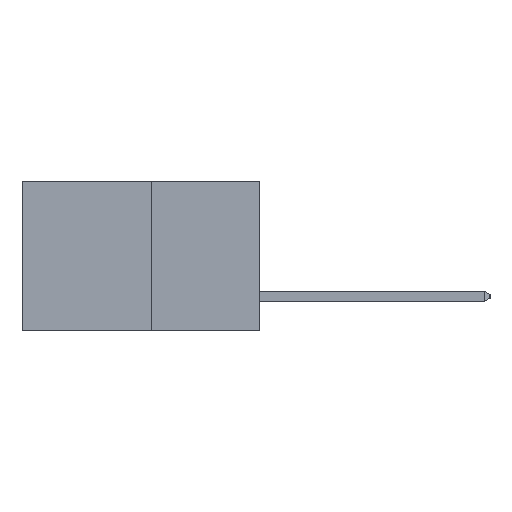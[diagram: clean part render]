
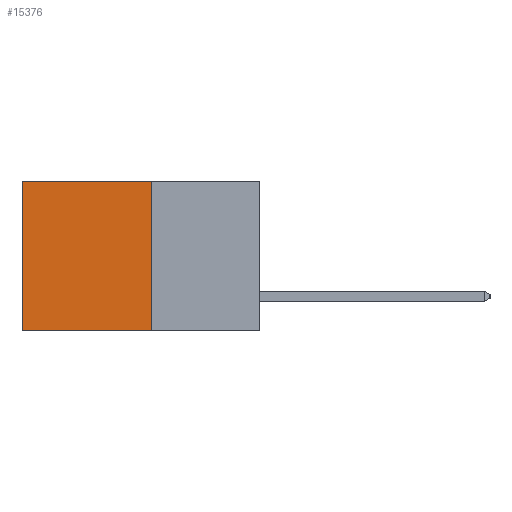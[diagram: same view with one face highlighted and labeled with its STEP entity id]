
A CAD part, left-side view. The second image highlights one B-rep face of the part: STEP entity #15376.
In plain terms, the highlighted planar face has unit normal (-1, 0, 0).
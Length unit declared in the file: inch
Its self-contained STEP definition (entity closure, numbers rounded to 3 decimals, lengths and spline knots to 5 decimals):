
#462 = DIRECTION ( 'NONE',  ( 1., 0., 0. ) ) ;
#981 = FACE_OUTER_BOUND ( 'NONE', #1252, .T. ) ;
#1162 = ORIENTED_EDGE ( 'NONE', *, *, #2322, .F. ) ;
#1252 = EDGE_LOOP ( 'NONE', ( #25020, #1162, #8642, #13474 ) ) ;
#1768 = EDGE_CURVE ( 'NONE', #18095, #10047, #10120, .T. ) ;
#2322 = EDGE_CURVE ( 'NONE', #16905, #10047, #8441, .T. ) ;
#2835 = DIRECTION ( 'NONE',  ( 0., 1., 0. ) ) ;
#3759 = CARTESIAN_POINT ( 'NONE',  ( 0.277, 0.27, -0.37 ) ) ;
#3883 = CARTESIAN_POINT ( 'NONE',  ( 0.277, 0.59, -0.37 ) ) ;
#4670 = VECTOR ( 'NONE', #23691, 39.37008 ) ;
#6234 = CARTESIAN_POINT ( 'NONE',  ( 0.277, 0.27, -0.37 ) ) ;
#6694 = VECTOR ( 'NONE', #22803, 39.37008 ) ;
#8441 = LINE ( 'NONE', #6234, #13174 ) ;
#8642 = ORIENTED_EDGE ( 'NONE', *, *, #23552, .F. ) ;
#8658 = CARTESIAN_POINT ( 'NONE',  ( 0.277, 0.59, -0.37 ) ) ;
#8874 = CARTESIAN_POINT ( 'NONE',  ( 0.277, 0.27, 0. ) ) ;
#9482 = VECTOR ( 'NONE', #9560, 39.37008 ) ;
#9560 = DIRECTION ( 'NONE',  ( 0., 0., -1. ) ) ;
#10047 = VERTEX_POINT ( 'NONE', #8658 ) ;
#10120 = LINE ( 'NONE', #3883, #9482 ) ;
#12476 = CARTESIAN_POINT ( 'NONE',  ( 0.277, 0.27, -0.37 ) ) ;
#13174 = VECTOR ( 'NONE', #2835, 39.37008 ) ;
#13474 = ORIENTED_EDGE ( 'NONE', *, *, #19857, .T. ) ;
#14497 = DIRECTION ( 'NONE',  ( 0., 0., -1. ) ) ;
#15300 = CARTESIAN_POINT ( 'NONE',  ( 0.277, 0.27, -0.37 ) ) ;
#15376 = ADVANCED_FACE ( 'NONE', ( #981 ), #18426, .F. ) ;
#15574 = CARTESIAN_POINT ( 'NONE',  ( 0.277, 0.27, 0. ) ) ;
#16905 = VERTEX_POINT ( 'NONE', #15300 ) ;
#18018 = LINE ( 'NONE', #8874, #6694 ) ;
#18095 = VERTEX_POINT ( 'NONE', #22764 ) ;
#18426 = PLANE ( 'NONE',  #22754 ) ;
#19857 = EDGE_CURVE ( 'NONE', #21324, #18095, #18018, .T. ) ;
#21221 = LINE ( 'NONE', #3759, #4670 ) ;
#21324 = VERTEX_POINT ( 'NONE', #15574 ) ;
#22754 = AXIS2_PLACEMENT_3D ( 'NONE', #12476, #462, #14497 ) ;
#22764 = CARTESIAN_POINT ( 'NONE',  ( 0.277, 0.59, 0. ) ) ;
#22803 = DIRECTION ( 'NONE',  ( 0., 1., 0. ) ) ;
#23552 = EDGE_CURVE ( 'NONE', #21324, #16905, #21221, .T. ) ;
#23691 = DIRECTION ( 'NONE',  ( 0., 0., -1. ) ) ;
#25020 = ORIENTED_EDGE ( 'NONE', *, *, #1768, .T. ) ;
